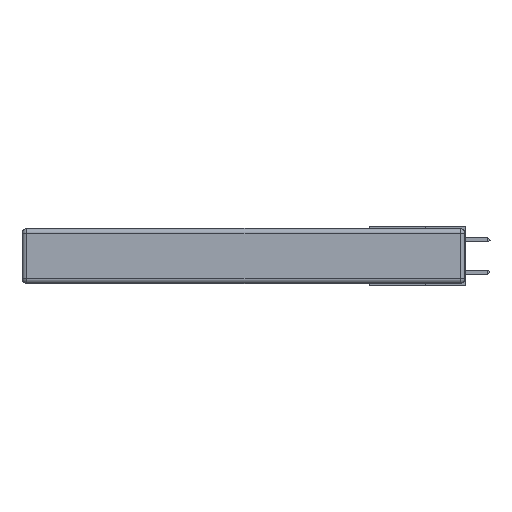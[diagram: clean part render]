
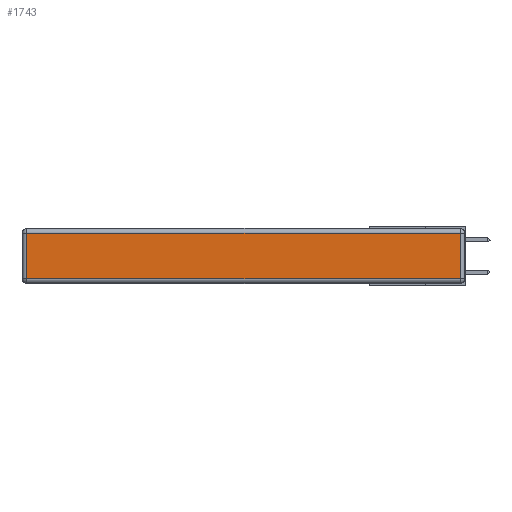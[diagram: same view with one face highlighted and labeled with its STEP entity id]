
A CAD part, left-side view. The second image highlights one B-rep face of the part: STEP entity #1743.
In plain terms, the highlighted planar face has unit normal (-1, 0, 0).
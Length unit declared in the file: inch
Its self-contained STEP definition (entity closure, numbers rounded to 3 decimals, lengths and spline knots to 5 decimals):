
#45 = VECTOR ( 'NONE', #24082, 39.37008 ) ;
#258 = CARTESIAN_POINT ( 'NONE',  ( 0., 0.03, -0.343 ) ) ;
#780 = ORIENTED_EDGE ( 'NONE', *, *, #4334, .T. ) ;
#1570 = VERTEX_POINT ( 'NONE', #10899 ) ;
#1650 = LINE ( 'NONE', #16927, #22628 ) ;
#1743 = ADVANCED_FACE ( 'NONE', ( #10365 ), #21116, .T. ) ;
#3522 = LINE ( 'NONE', #258, #23566 ) ;
#4334 = EDGE_CURVE ( 'NONE', #1570, #17301, #1650, .T. ) ;
#4875 = DIRECTION ( 'NONE',  ( -1., 0., 0. ) ) ;
#5725 = VECTOR ( 'NONE', #16019, 39.37008 ) ;
#9787 = CARTESIAN_POINT ( 'NONE',  ( 0., 0.03, -0.03 ) ) ;
#10365 = FACE_OUTER_BOUND ( 'NONE', #20371, .T. ) ;
#10814 = DIRECTION ( 'NONE',  ( 0., 0., -1. ) ) ;
#10899 = CARTESIAN_POINT ( 'NONE',  ( 0., 2.72, -0.03 ) ) ;
#10902 = LINE ( 'NONE', #15720, #45 ) ;
#11015 = CARTESIAN_POINT ( 'NONE',  ( 0., 2.72, -0.313 ) ) ;
#11177 = CARTESIAN_POINT ( 'NONE',  ( 0., 0.03, -0.313 ) ) ;
#11481 = LINE ( 'NONE', #24047, #5725 ) ;
#12565 = DIRECTION ( 'NONE',  ( 0., 0., 1. ) ) ;
#13081 = CARTESIAN_POINT ( 'NONE',  ( 0., 0., -0.343 ) ) ;
#14773 = EDGE_CURVE ( 'NONE', #17301, #17831, #10902, .T. ) ;
#15720 = CARTESIAN_POINT ( 'NONE',  ( 0., 0., -0.313 ) ) ;
#16019 = DIRECTION ( 'NONE',  ( 0., 1., 0. ) ) ;
#16927 = CARTESIAN_POINT ( 'NONE',  ( 0., 2.72, -0.343 ) ) ;
#17050 = ORIENTED_EDGE ( 'NONE', *, *, #22978, .T. ) ;
#17301 = VERTEX_POINT ( 'NONE', #11015 ) ;
#17831 = VERTEX_POINT ( 'NONE', #11177 ) ;
#17964 = EDGE_CURVE ( 'NONE', #17831, #18281, #3522, .T. ) ;
#18281 = VERTEX_POINT ( 'NONE', #9787 ) ;
#20371 = EDGE_LOOP ( 'NONE', ( #20591, #25443, #17050, #780 ) ) ;
#20591 = ORIENTED_EDGE ( 'NONE', *, *, #14773, .T. ) ;
#21116 = PLANE ( 'NONE',  #21733 ) ;
#21733 = AXIS2_PLACEMENT_3D ( 'NONE', #13081, #4875, #25112 ) ;
#22628 = VECTOR ( 'NONE', #10814, 39.37008 ) ;
#22978 = EDGE_CURVE ( 'NONE', #18281, #1570, #11481, .T. ) ;
#23566 = VECTOR ( 'NONE', #12565, 39.37008 ) ;
#24047 = CARTESIAN_POINT ( 'NONE',  ( 0., 2.75, -0.03 ) ) ;
#24082 = DIRECTION ( 'NONE',  ( 0., -1., 0. ) ) ;
#25112 = DIRECTION ( 'NONE',  ( 0., 0., 1. ) ) ;
#25443 = ORIENTED_EDGE ( 'NONE', *, *, #17964, .T. ) ;
